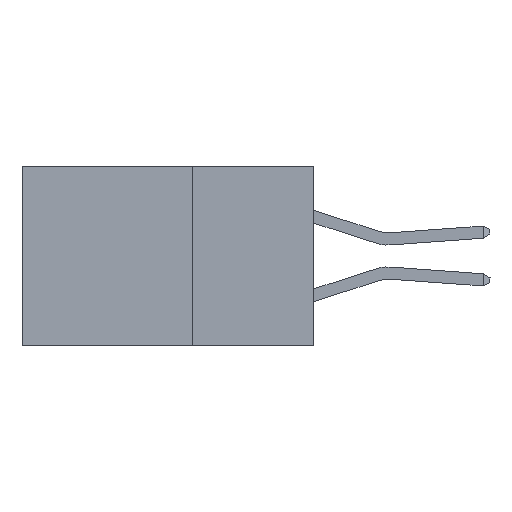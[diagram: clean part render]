
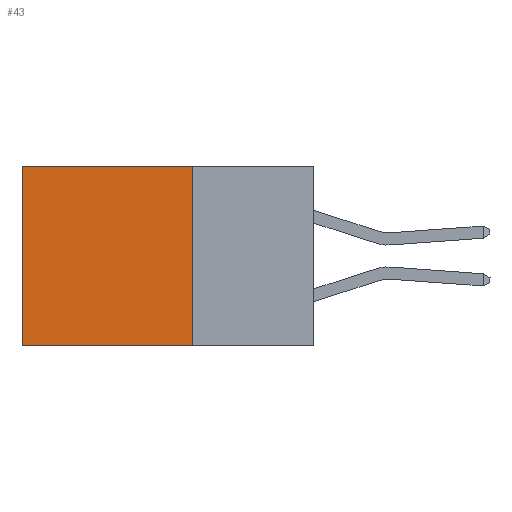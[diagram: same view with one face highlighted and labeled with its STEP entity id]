
A CAD part, left-side view. The second image highlights one B-rep face of the part: STEP entity #43.
In plain terms, the highlighted planar face has unit normal (-1, 0, 0).
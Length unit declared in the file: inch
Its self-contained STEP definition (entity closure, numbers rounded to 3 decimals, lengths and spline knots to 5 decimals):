
#43 = ADVANCED_FACE ( 'NONE', ( #16313 ), #17421, .F. ) ;
#447 = VERTEX_POINT ( 'NONE', #19156 ) ;
#503 = CARTESIAN_POINT ( 'NONE',  ( 0.2875, 0.6, -0.37 ) ) ;
#1003 = CARTESIAN_POINT ( 'NONE',  ( 0.2875, 0.25, 0. ) ) ;
#1920 = ORIENTED_EDGE ( 'NONE', *, *, #17365, .T. ) ;
#2154 = VERTEX_POINT ( 'NONE', #13529 ) ;
#2247 = CARTESIAN_POINT ( 'NONE',  ( 0.2875, 0.25, -0.37 ) ) ;
#2317 = DIRECTION ( 'NONE',  ( 0., 0., -1. ) ) ;
#2906 = EDGE_CURVE ( 'NONE', #2154, #14774, #16921, .T. ) ;
#4178 = LINE ( 'NONE', #11333, #18983 ) ;
#4564 = EDGE_LOOP ( 'NONE', ( #18552, #10650, #17458, #1920 ) ) ;
#4971 = DIRECTION ( 'NONE',  ( 0., 1., 0. ) ) ;
#6451 = DIRECTION ( 'NONE',  ( 0., 0., -1. ) ) ;
#7734 = LINE ( 'NONE', #13934, #15621 ) ;
#8624 = LINE ( 'NONE', #14545, #12619 ) ;
#10547 = DIRECTION ( 'NONE',  ( 1., 0., 0. ) ) ;
#10650 = ORIENTED_EDGE ( 'NONE', *, *, #18855, .F. ) ;
#11333 = CARTESIAN_POINT ( 'NONE',  ( 0.2875, 0.25, 0. ) ) ;
#12619 = VECTOR ( 'NONE', #14600, 39.37008 ) ;
#13499 = VECTOR ( 'NONE', #6451, 39.37008 ) ;
#13529 = CARTESIAN_POINT ( 'NONE',  ( 0.2875, 0.6, 0. ) ) ;
#13832 = VERTEX_POINT ( 'NONE', #2247 ) ;
#13934 = CARTESIAN_POINT ( 'NONE',  ( 0.2875, 0.25, 0. ) ) ;
#14541 = AXIS2_PLACEMENT_3D ( 'NONE', #1003, #10547, #17208 ) ;
#14545 = CARTESIAN_POINT ( 'NONE',  ( 0.2875, 0.25, -0.37 ) ) ;
#14600 = DIRECTION ( 'NONE',  ( 0., 1., 0. ) ) ;
#14774 = VERTEX_POINT ( 'NONE', #503 ) ;
#15621 = VECTOR ( 'NONE', #4971, 39.37008 ) ;
#16313 = FACE_OUTER_BOUND ( 'NONE', #4564, .T. ) ;
#16819 = CARTESIAN_POINT ( 'NONE',  ( 0.2875, 0.6, 0. ) ) ;
#16921 = LINE ( 'NONE', #16819, #13499 ) ;
#17208 = DIRECTION ( 'NONE',  ( 0., 0., -1. ) ) ;
#17365 = EDGE_CURVE ( 'NONE', #447, #2154, #7734, .T. ) ;
#17421 = PLANE ( 'NONE',  #14541 ) ;
#17458 = ORIENTED_EDGE ( 'NONE', *, *, #18077, .F. ) ;
#18077 = EDGE_CURVE ( 'NONE', #447, #13832, #4178, .T. ) ;
#18552 = ORIENTED_EDGE ( 'NONE', *, *, #2906, .T. ) ;
#18855 = EDGE_CURVE ( 'NONE', #13832, #14774, #8624, .T. ) ;
#18983 = VECTOR ( 'NONE', #2317, 39.37008 ) ;
#19156 = CARTESIAN_POINT ( 'NONE',  ( 0.2875, 0.25, 0. ) ) ;
